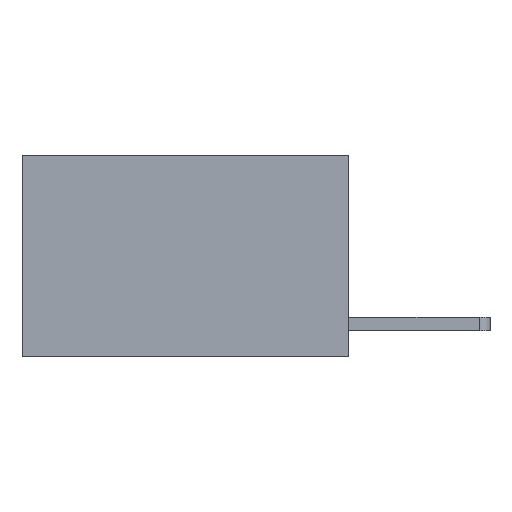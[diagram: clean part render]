
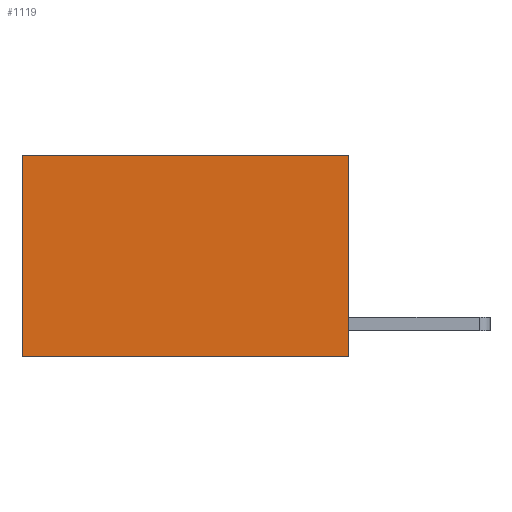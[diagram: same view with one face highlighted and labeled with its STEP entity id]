
A CAD part, left-side view. The second image highlights one B-rep face of the part: STEP entity #1119.
In plain terms, the highlighted planar face has unit normal (-1, 0, 0).
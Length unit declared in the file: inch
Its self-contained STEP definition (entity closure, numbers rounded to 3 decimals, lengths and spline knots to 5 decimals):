
#179 = LINE ( 'NONE', #4018, #1743 ) ;
#442 = CARTESIAN_POINT ( 'NONE',  ( 0.2625, 0., -0.37 ) ) ;
#465 = VECTOR ( 'NONE', #1820, 39.37008 ) ;
#622 = ORIENTED_EDGE ( 'NONE', *, *, #7395, .F. ) ;
#655 = LINE ( 'NONE', #4197, #465 ) ;
#716 = DIRECTION ( 'NONE',  ( 0., 0., -1. ) ) ;
#775 = EDGE_LOOP ( 'NONE', ( #5236, #3793, #622, #4517 ) ) ;
#1119 = ADVANCED_FACE ( 'NONE', ( #3832 ), #6471, .F. ) ;
#1743 = VECTOR ( 'NONE', #2811, 39.37008 ) ;
#1820 = DIRECTION ( 'NONE',  ( 0., 1., 0. ) ) ;
#1966 = VECTOR ( 'NONE', #716, 39.37008 ) ;
#2155 = DIRECTION ( 'NONE',  ( 0., 0., -1. ) ) ;
#2724 = EDGE_CURVE ( 'NONE', #6808, #4784, #655, .T. ) ;
#2811 = DIRECTION ( 'NONE',  ( 0., 1., 0. ) ) ;
#3175 = VERTEX_POINT ( 'NONE', #5562 ) ;
#3494 = DIRECTION ( 'NONE',  ( 0., 0., -1. ) ) ;
#3793 = ORIENTED_EDGE ( 'NONE', *, *, #2724, .F. ) ;
#3832 = FACE_OUTER_BOUND ( 'NONE', #775, .T. ) ;
#4018 = CARTESIAN_POINT ( 'NONE',  ( 0.2625, 0., 0. ) ) ;
#4080 = EDGE_CURVE ( 'NONE', #3175, #5713, #179, .T. ) ;
#4197 = CARTESIAN_POINT ( 'NONE',  ( 0.2625, 0., -0.37 ) ) ;
#4264 = CARTESIAN_POINT ( 'NONE',  ( 0.2625, 0.6, 0. ) ) ;
#4301 = CARTESIAN_POINT ( 'NONE',  ( 0.2625, 0.6, 0. ) ) ;
#4501 = AXIS2_PLACEMENT_3D ( 'NONE', #7673, #7090, #3494 ) ;
#4517 = ORIENTED_EDGE ( 'NONE', *, *, #4080, .T. ) ;
#4784 = VERTEX_POINT ( 'NONE', #5635 ) ;
#5150 = CARTESIAN_POINT ( 'NONE',  ( 0.2625, 0., 0. ) ) ;
#5236 = ORIENTED_EDGE ( 'NONE', *, *, #7068, .T. ) ;
#5562 = CARTESIAN_POINT ( 'NONE',  ( 0.2625, 0., 0. ) ) ;
#5635 = CARTESIAN_POINT ( 'NONE',  ( 0.2625, 0.6, -0.37 ) ) ;
#5713 = VERTEX_POINT ( 'NONE', #4264 ) ;
#6124 = LINE ( 'NONE', #5150, #6296 ) ;
#6296 = VECTOR ( 'NONE', #2155, 39.37008 ) ;
#6471 = PLANE ( 'NONE',  #4501 ) ;
#6532 = LINE ( 'NONE', #4301, #1966 ) ;
#6808 = VERTEX_POINT ( 'NONE', #442 ) ;
#7068 = EDGE_CURVE ( 'NONE', #5713, #4784, #6532, .T. ) ;
#7090 = DIRECTION ( 'NONE',  ( 1., 0., 0. ) ) ;
#7395 = EDGE_CURVE ( 'NONE', #3175, #6808, #6124, .T. ) ;
#7673 = CARTESIAN_POINT ( 'NONE',  ( 0.2625, 0., 0. ) ) ;
